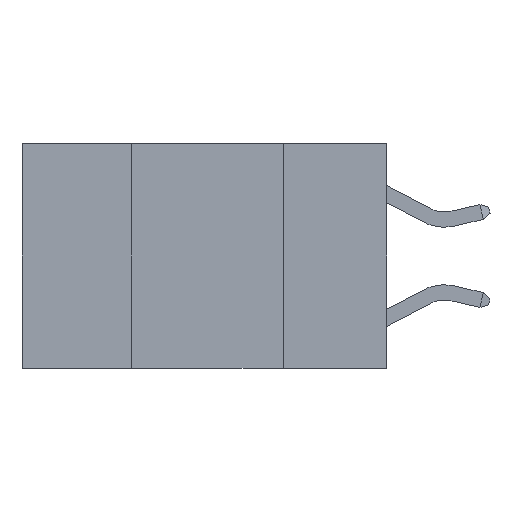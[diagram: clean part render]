
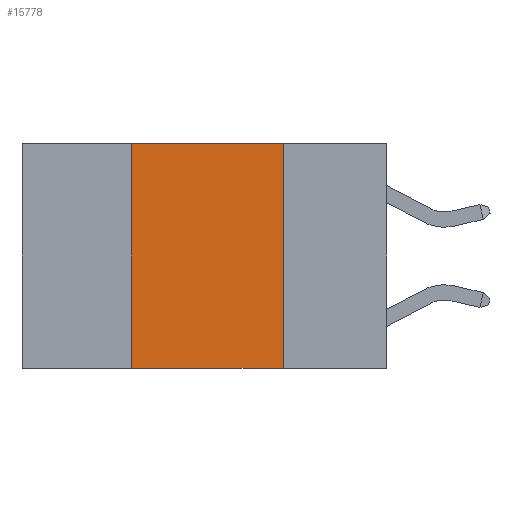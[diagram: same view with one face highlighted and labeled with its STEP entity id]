
A CAD part, left-side view. The second image highlights one B-rep face of the part: STEP entity #15778.
In plain terms, the highlighted planar face has unit normal (-1, 0, 0).
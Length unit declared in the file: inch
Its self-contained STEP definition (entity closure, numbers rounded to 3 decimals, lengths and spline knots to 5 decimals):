
#100 = DIRECTION ( 'NONE',  ( 0., 0., -1. ) ) ;
#903 = VERTEX_POINT ( 'NONE', #13973 ) ;
#1825 = CARTESIAN_POINT ( 'NONE',  ( 0., 0.6, -0.37 ) ) ;
#3369 = DIRECTION ( 'NONE',  ( 0., 0., -1. ) ) ;
#5211 = EDGE_LOOP ( 'NONE', ( #17461, #7667, #5511, #16895 ) ) ;
#5511 = ORIENTED_EDGE ( 'NONE', *, *, #17916, .F. ) ;
#6002 = CARTESIAN_POINT ( 'NONE',  ( 0., 0.42, -0.37 ) ) ;
#6149 = LINE ( 'NONE', #1825, #18506 ) ;
#6341 = PLANE ( 'NONE',  #17389 ) ;
#7262 = LINE ( 'NONE', #16451, #19157 ) ;
#7667 = ORIENTED_EDGE ( 'NONE', *, *, #18726, .F. ) ;
#7918 = CARTESIAN_POINT ( 'NONE',  ( 0., 0.6, 0. ) ) ;
#7925 = VERTEX_POINT ( 'NONE', #11237 ) ;
#8457 = VECTOR ( 'NONE', #3369, 39.37008 ) ;
#8458 = VERTEX_POINT ( 'NONE', #12052 ) ;
#9485 = DIRECTION ( 'NONE',  ( 1., 0., 0. ) ) ;
#11130 = CARTESIAN_POINT ( 'NONE',  ( 0., 0.17, 0. ) ) ;
#11237 = CARTESIAN_POINT ( 'NONE',  ( 0., 0.42, 0. ) ) ;
#11745 = FACE_OUTER_BOUND ( 'NONE', #5211, .T. ) ;
#12052 = CARTESIAN_POINT ( 'NONE',  ( 0., 0.17, -0.37 ) ) ;
#12144 = DIRECTION ( 'NONE',  ( 0., -1., 0. ) ) ;
#12727 = DIRECTION ( 'NONE',  ( 0., -1., 0. ) ) ;
#12822 = VECTOR ( 'NONE', #12144, 39.37008 ) ;
#13973 = CARTESIAN_POINT ( 'NONE',  ( 0., 0.17, 0. ) ) ;
#14085 = VERTEX_POINT ( 'NONE', #6002 ) ;
#14917 = DIRECTION ( 'NONE',  ( 0., 0., 1. ) ) ;
#15778 = ADVANCED_FACE ( 'NONE', ( #11745 ), #6341, .F. ) ;
#15825 = EDGE_CURVE ( 'NONE', #14085, #8458, #6149, .T. ) ;
#16451 = CARTESIAN_POINT ( 'NONE',  ( 0., 0.42, 0. ) ) ;
#16653 = LINE ( 'NONE', #11130, #8457 ) ;
#16895 = ORIENTED_EDGE ( 'NONE', *, *, #15825, .T. ) ;
#17389 = AXIS2_PLACEMENT_3D ( 'NONE', #7918, #9485, #100 ) ;
#17409 = LINE ( 'NONE', #18273, #12822 ) ;
#17461 = ORIENTED_EDGE ( 'NONE', *, *, #18967, .F. ) ;
#17916 = EDGE_CURVE ( 'NONE', #14085, #7925, #7262, .T. ) ;
#18273 = CARTESIAN_POINT ( 'NONE',  ( 0., 0.6, 0. ) ) ;
#18506 = VECTOR ( 'NONE', #12727, 39.37008 ) ;
#18726 = EDGE_CURVE ( 'NONE', #7925, #903, #17409, .T. ) ;
#18967 = EDGE_CURVE ( 'NONE', #903, #8458, #16653, .T. ) ;
#19157 = VECTOR ( 'NONE', #14917, 39.37008 ) ;
